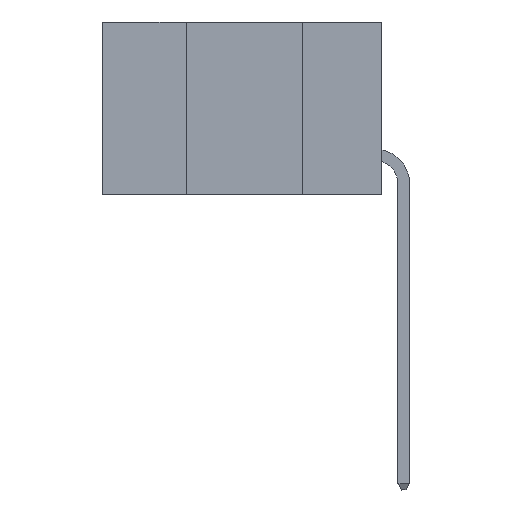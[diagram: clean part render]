
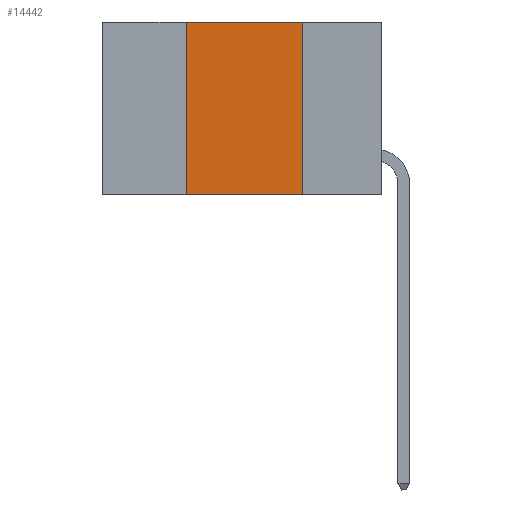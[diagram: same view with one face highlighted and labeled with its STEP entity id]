
A CAD part, left-side view. The second image highlights one B-rep face of the part: STEP entity #14442.
In plain terms, the highlighted planar face has unit normal (-1, 0, 0).
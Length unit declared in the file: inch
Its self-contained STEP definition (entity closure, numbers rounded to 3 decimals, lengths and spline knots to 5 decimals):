
#13 = VECTOR ( 'NONE', #2581, 39.37008 ) ;
#811 = LINE ( 'NONE', #12937, #21260 ) ;
#1200 = DIRECTION ( 'NONE',  ( 0., 0., -1. ) ) ;
#1264 = VECTOR ( 'NONE', #1200, 39.37008 ) ;
#1390 = VERTEX_POINT ( 'NONE', #23464 ) ;
#2581 = DIRECTION ( 'NONE',  ( 0., -1., 0. ) ) ;
#2605 = ORIENTED_EDGE ( 'NONE', *, *, #24876, .F. ) ;
#2658 = CARTESIAN_POINT ( 'NONE',  ( 0., 0.6, 0. ) ) ;
#4482 = VERTEX_POINT ( 'NONE', #13251 ) ;
#5176 = DIRECTION ( 'NONE',  ( 0., -1., 0. ) ) ;
#6372 = DIRECTION ( 'NONE',  ( 1., 0., 0. ) ) ;
#6981 = DIRECTION ( 'NONE',  ( 0., 0., 1. ) ) ;
#7148 = VECTOR ( 'NONE', #5176, 39.37008 ) ;
#7964 = EDGE_CURVE ( 'NONE', #1390, #25130, #811, .T. ) ;
#8112 = DIRECTION ( 'NONE',  ( 0., 0., -1. ) ) ;
#8208 = CARTESIAN_POINT ( 'NONE',  ( 0., 0.42, 0. ) ) ;
#8656 = ORIENTED_EDGE ( 'NONE', *, *, #7964, .F. ) ;
#9325 = CARTESIAN_POINT ( 'NONE',  ( 0., 0.17, 0. ) ) ;
#11087 = EDGE_CURVE ( 'NONE', #25130, #4482, #22615, .T. ) ;
#11151 = LINE ( 'NONE', #9325, #1264 ) ;
#12279 = AXIS2_PLACEMENT_3D ( 'NONE', #18201, #6372, #8112 ) ;
#12937 = CARTESIAN_POINT ( 'NONE',  ( 0., 0.42, 0. ) ) ;
#13251 = CARTESIAN_POINT ( 'NONE',  ( 0., 0.17, 0. ) ) ;
#14442 = ADVANCED_FACE ( 'NONE', ( #14742 ), #24017, .F. ) ;
#14603 = ORIENTED_EDGE ( 'NONE', *, *, #11087, .F. ) ;
#14742 = FACE_OUTER_BOUND ( 'NONE', #24326, .T. ) ;
#17658 = ORIENTED_EDGE ( 'NONE', *, *, #24867, .T. ) ;
#18201 = CARTESIAN_POINT ( 'NONE',  ( 0., 0.6, 0. ) ) ;
#19159 = CARTESIAN_POINT ( 'NONE',  ( 0., 0.6, -0.37 ) ) ;
#19654 = CARTESIAN_POINT ( 'NONE',  ( 0., 0.17, -0.37 ) ) ;
#21260 = VECTOR ( 'NONE', #6981, 39.37008 ) ;
#21721 = LINE ( 'NONE', #19159, #7148 ) ;
#22615 = LINE ( 'NONE', #2658, #13 ) ;
#23448 = VERTEX_POINT ( 'NONE', #19654 ) ;
#23464 = CARTESIAN_POINT ( 'NONE',  ( 0., 0.42, -0.37 ) ) ;
#24017 = PLANE ( 'NONE',  #12279 ) ;
#24326 = EDGE_LOOP ( 'NONE', ( #2605, #14603, #8656, #17658 ) ) ;
#24867 = EDGE_CURVE ( 'NONE', #1390, #23448, #21721, .T. ) ;
#24876 = EDGE_CURVE ( 'NONE', #4482, #23448, #11151, .T. ) ;
#25130 = VERTEX_POINT ( 'NONE', #8208 ) ;
